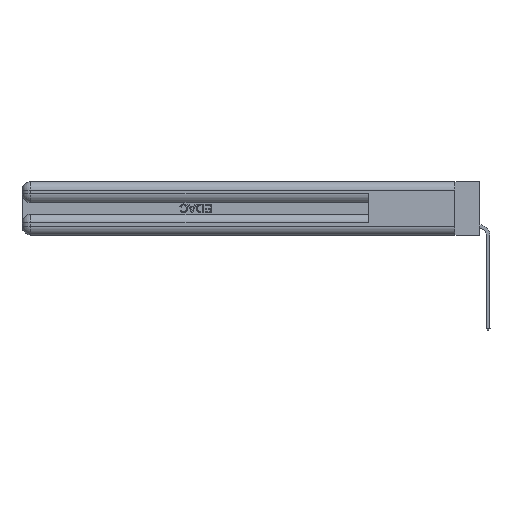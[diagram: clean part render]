
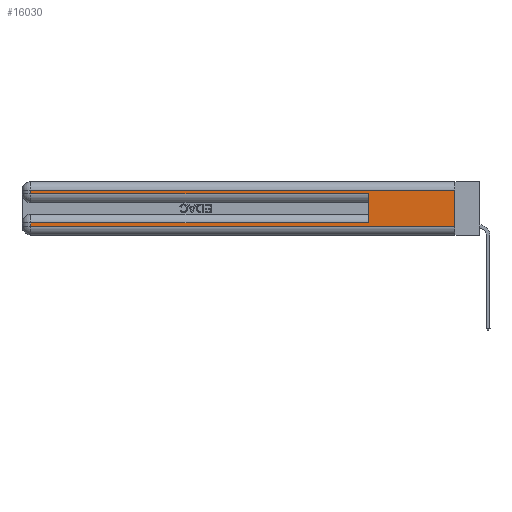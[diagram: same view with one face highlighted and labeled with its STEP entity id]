
A CAD part, left-side view. The second image highlights one B-rep face of the part: STEP entity #16030.
In plain terms, the highlighted planar face has unit normal (-1, 0, 0).
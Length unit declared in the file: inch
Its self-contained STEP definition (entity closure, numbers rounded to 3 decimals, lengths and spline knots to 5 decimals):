
#788 = VERTEX_POINT ( 'NONE', #3561 ) ;
#857 = AXIS2_PLACEMENT_3D ( 'NONE', #18553, #16412, #18697 ) ;
#1250 = CARTESIAN_POINT ( 'NONE',  ( 0., 0., 0.085 ) ) ;
#1608 = VECTOR ( 'NONE', #11505, 39.37008 ) ;
#2056 = DIRECTION ( 'NONE',  ( 0., 0., -1. ) ) ;
#2843 = ORIENTED_EDGE ( 'NONE', *, *, #9655, .T. ) ;
#2883 = DIRECTION ( 'NONE',  ( 0., -1., 0. ) ) ;
#2894 = LINE ( 'NONE', #12839, #21608 ) ;
#2956 = ORIENTED_EDGE ( 'NONE', *, *, #9987, .T. ) ;
#2969 = VERTEX_POINT ( 'NONE', #12563 ) ;
#3561 = CARTESIAN_POINT ( 'NONE',  ( 0., 0., 0.31 ) ) ;
#4529 = CARTESIAN_POINT ( 'NONE',  ( 0., 2.94, 0.285 ) ) ;
#4807 = LINE ( 'NONE', #23926, #1608 ) ;
#5228 = EDGE_CURVE ( 'NONE', #788, #31684, #4807, .T. ) ;
#6186 = CARTESIAN_POINT ( 'NONE',  ( 0., 0.6, 0.085 ) ) ;
#6307 = VERTEX_POINT ( 'NONE', #10238 ) ;
#6615 = CARTESIAN_POINT ( 'NONE',  ( 0., 2.94, 0.085 ) ) ;
#6673 = LINE ( 'NONE', #22024, #20460 ) ;
#6907 = CARTESIAN_POINT ( 'NONE',  ( 0., 0., 0.31 ) ) ;
#7031 = ORIENTED_EDGE ( 'NONE', *, *, #22001, .F. ) ;
#7176 = CARTESIAN_POINT ( 'NONE',  ( 0., 2.94, 0.37 ) ) ;
#7228 = DIRECTION ( 'NONE',  ( 0., 1., 0. ) ) ;
#7330 = EDGE_CURVE ( 'NONE', #788, #2969, #11966, .T. ) ;
#9005 = ORIENTED_EDGE ( 'NONE', *, *, #18872, .T. ) ;
#9249 = ORIENTED_EDGE ( 'NONE', *, *, #27687, .T. ) ;
#9655 = EDGE_CURVE ( 'NONE', #11669, #28411, #13993, .T. ) ;
#9987 = EDGE_CURVE ( 'NONE', #26163, #6307, #2894, .T. ) ;
#10238 = CARTESIAN_POINT ( 'NONE',  ( 0., 0.6, 0.285 ) ) ;
#10440 = ORIENTED_EDGE ( 'NONE', *, *, #5228, .F. ) ;
#11226 = DIRECTION ( 'NONE',  ( 0., 1., 0. ) ) ;
#11307 = ORIENTED_EDGE ( 'NONE', *, *, #7330, .T. ) ;
#11505 = DIRECTION ( 'NONE',  ( 0., 0., -1. ) ) ;
#11669 = VERTEX_POINT ( 'NONE', #6186 ) ;
#11966 = LINE ( 'NONE', #6907, #25792 ) ;
#12563 = CARTESIAN_POINT ( 'NONE',  ( 0., 2.94, 0.31 ) ) ;
#12839 = CARTESIAN_POINT ( 'NONE',  ( 0., 0., 0.285 ) ) ;
#13993 = LINE ( 'NONE', #1250, #31586 ) ;
#14973 = LINE ( 'NONE', #25114, #18378 ) ;
#15777 = FACE_OUTER_BOUND ( 'NONE', #21338, .T. ) ;
#15936 = ORIENTED_EDGE ( 'NONE', *, *, #24636, .T. ) ;
#16030 = ADVANCED_FACE ( 'NONE', ( #15777 ), #28860, .F. ) ;
#16412 = DIRECTION ( 'NONE',  ( 1., 0., 0. ) ) ;
#17574 = CARTESIAN_POINT ( 'NONE',  ( 0., 2.94, 0.06 ) ) ;
#18378 = VECTOR ( 'NONE', #2056, 39.37008 ) ;
#18553 = CARTESIAN_POINT ( 'NONE',  ( 0., 0., 0.37 ) ) ;
#18697 = DIRECTION ( 'NONE',  ( 0., 0., -1. ) ) ;
#18872 = EDGE_CURVE ( 'NONE', #2969, #26163, #14973, .T. ) ;
#20460 = VECTOR ( 'NONE', #22197, 39.37008 ) ;
#21338 = EDGE_LOOP ( 'NONE', ( #10440, #11307, #9005, #2956, #7031, #2843, #9249, #15936 ) ) ;
#21608 = VECTOR ( 'NONE', #25454, 39.37008 ) ;
#21726 = LINE ( 'NONE', #7176, #29528 ) ;
#22001 = EDGE_CURVE ( 'NONE', #11669, #6307, #6673, .T. ) ;
#22024 = CARTESIAN_POINT ( 'NONE',  ( 0., 0.6, 0.145 ) ) ;
#22197 = DIRECTION ( 'NONE',  ( 0., 0., 1. ) ) ;
#22992 = LINE ( 'NONE', #23138, #32094 ) ;
#23138 = CARTESIAN_POINT ( 'NONE',  ( 0., 0., 0.06 ) ) ;
#23926 = CARTESIAN_POINT ( 'NONE',  ( 0., 0., 0.37 ) ) ;
#24636 = EDGE_CURVE ( 'NONE', #28607, #31684, #22992, .T. ) ;
#25114 = CARTESIAN_POINT ( 'NONE',  ( 0., 2.94, 0.37 ) ) ;
#25454 = DIRECTION ( 'NONE',  ( 0., -1., 0. ) ) ;
#25792 = VECTOR ( 'NONE', #7228, 39.37008 ) ;
#26163 = VERTEX_POINT ( 'NONE', #4529 ) ;
#27687 = EDGE_CURVE ( 'NONE', #28411, #28607, #21726, .T. ) ;
#28411 = VERTEX_POINT ( 'NONE', #6615 ) ;
#28607 = VERTEX_POINT ( 'NONE', #17574 ) ;
#28860 = PLANE ( 'NONE',  #857 ) ;
#29528 = VECTOR ( 'NONE', #31748, 39.37008 ) ;
#29894 = CARTESIAN_POINT ( 'NONE',  ( 0., 0., 0.06 ) ) ;
#31586 = VECTOR ( 'NONE', #11226, 39.37008 ) ;
#31684 = VERTEX_POINT ( 'NONE', #29894 ) ;
#31748 = DIRECTION ( 'NONE',  ( 0., 0., -1. ) ) ;
#32094 = VECTOR ( 'NONE', #2883, 39.37008 ) ;
